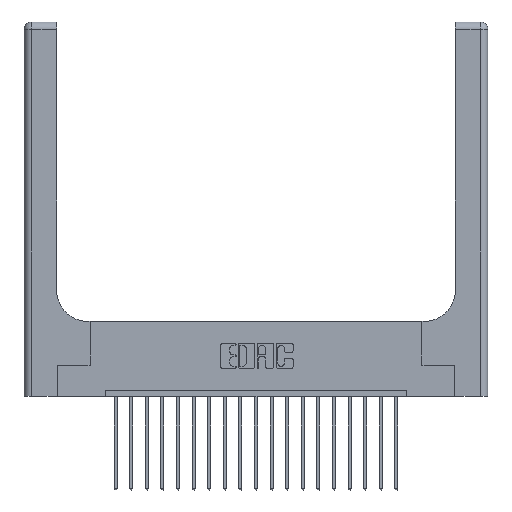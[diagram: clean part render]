
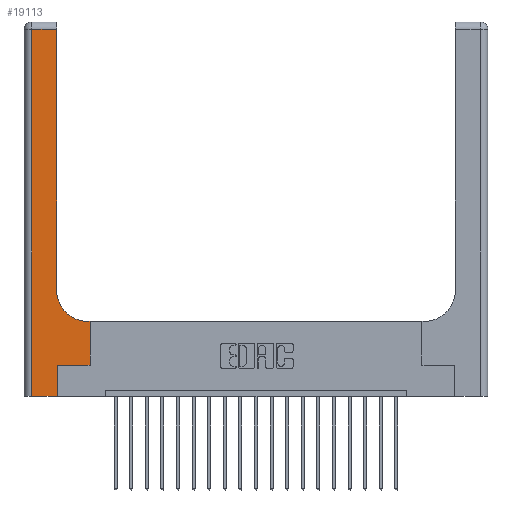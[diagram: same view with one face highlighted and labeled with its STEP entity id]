
A CAD part, top view. The second image highlights one B-rep face of the part: STEP entity #19113.
In plain terms, the highlighted planar face has unit normal (0, 0, 1).
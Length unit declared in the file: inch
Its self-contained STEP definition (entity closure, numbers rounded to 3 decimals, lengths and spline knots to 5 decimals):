
#205 = VERTEX_POINT ( 'NONE', #5809 ) ;
#565 = ORIENTED_EDGE ( 'NONE', *, *, #14055, .T. ) ;
#1562 = PLANE ( 'NONE',  #1674 ) ;
#1574 = VERTEX_POINT ( 'NONE', #9446 ) ;
#1597 = ORIENTED_EDGE ( 'NONE', *, *, #5390, .T. ) ;
#1674 = AXIS2_PLACEMENT_3D ( 'NONE', #18800, #18998, #10796 ) ;
#1866 = VERTEX_POINT ( 'NONE', #15172 ) ;
#1882 = CARTESIAN_POINT ( 'NONE',  ( 0.26, 3., 0.37 ) ) ;
#1920 = CARTESIAN_POINT ( 'NONE',  ( 0.06, 3., 0.37 ) ) ;
#2401 = DIRECTION ( 'NONE',  ( 1., 0., 0. ) ) ;
#2470 = EDGE_CURVE ( 'NONE', #205, #1574, #20418, .T. ) ;
#2886 = CARTESIAN_POINT ( 'NONE',  ( 0.26, 2.94, 0.37 ) ) ;
#4099 = ORIENTED_EDGE ( 'NONE', *, *, #5455, .T. ) ;
#4237 = VECTOR ( 'NONE', #11684, 39.37008 ) ;
#4964 = CARTESIAN_POINT ( 'NONE',  ( 0.265, 0., 0.37 ) ) ;
#5390 = EDGE_CURVE ( 'NONE', #12642, #20198, #8114, .T. ) ;
#5455 = EDGE_CURVE ( 'NONE', #1574, #1866, #7078, .T. ) ;
#5692 = VECTOR ( 'NONE', #7021, 39.37008 ) ;
#5809 = CARTESIAN_POINT ( 'NONE',  ( 0.265, 0., 0.37 ) ) ;
#6081 = CARTESIAN_POINT ( 'NONE',  ( 0., 0., 0.37 ) ) ;
#6245 = EDGE_LOOP ( 'NONE', ( #1597, #9969, #10971, #14447, #13088, #4099, #565, #10019, #12078 ) ) ;
#7021 = DIRECTION ( 'NONE',  ( -1., 0., 0. ) ) ;
#7078 = LINE ( 'NONE', #11968, #18723 ) ;
#7241 = CIRCLE ( 'NONE', #13203, 0.25 ) ;
#7631 = LINE ( 'NONE', #6081, #19554 ) ;
#8114 = LINE ( 'NONE', #1882, #10755 ) ;
#9100 = VERTEX_POINT ( 'NONE', #10749 ) ;
#9446 = CARTESIAN_POINT ( 'NONE',  ( 0.265, 0.25, 0.37 ) ) ;
#9497 = DIRECTION ( 'NONE',  ( 0., 1., 0. ) ) ;
#9542 = FACE_OUTER_BOUND ( 'NONE', #6245, .T. ) ;
#9969 = ORIENTED_EDGE ( 'NONE', *, *, #15376, .T. ) ;
#10019 = ORIENTED_EDGE ( 'NONE', *, *, #19463, .T. ) ;
#10209 = VERTEX_POINT ( 'NONE', #19913 ) ;
#10443 = CARTESIAN_POINT ( 'NONE',  ( 0.26, 0.85, 0.37 ) ) ;
#10749 = CARTESIAN_POINT ( 'NONE',  ( 0.528, 0.6, 0.37 ) ) ;
#10755 = VECTOR ( 'NONE', #19226, 39.37008 ) ;
#10796 = DIRECTION ( 'NONE',  ( -1., 0., 0. ) ) ;
#10971 = ORIENTED_EDGE ( 'NONE', *, *, #12906, .T. ) ;
#11016 = VERTEX_POINT ( 'NONE', #13533 ) ;
#11166 = CARTESIAN_POINT ( 'NONE',  ( 0.528, 0.25, 0.37 ) ) ;
#11408 = VECTOR ( 'NONE', #9497, 39.37008 ) ;
#11684 = DIRECTION ( 'NONE',  ( -1., 0., 0. ) ) ;
#11692 = LINE ( 'NONE', #18029, #5692 ) ;
#11968 = CARTESIAN_POINT ( 'NONE',  ( 0.265, 0.25, 0.37 ) ) ;
#12078 = ORIENTED_EDGE ( 'NONE', *, *, #16099, .T. ) ;
#12175 = CARTESIAN_POINT ( 'NONE',  ( 0.51, 0.85, 0.37 ) ) ;
#12642 = VERTEX_POINT ( 'NONE', #10443 ) ;
#12906 = EDGE_CURVE ( 'NONE', #17054, #11016, #19358, .T. ) ;
#13088 = ORIENTED_EDGE ( 'NONE', *, *, #2470, .T. ) ;
#13203 = AXIS2_PLACEMENT_3D ( 'NONE', #12175, #20073, #19972 ) ;
#13252 = CARTESIAN_POINT ( 'NONE',  ( 0., 2.94, 0.37 ) ) ;
#13533 = CARTESIAN_POINT ( 'NONE',  ( 0.06, 0., 0.37 ) ) ;
#13882 = DIRECTION ( 'NONE',  ( 0., 1., 0. ) ) ;
#14055 = EDGE_CURVE ( 'NONE', #1866, #9100, #15648, .T. ) ;
#14447 = ORIENTED_EDGE ( 'NONE', *, *, #18237, .T. ) ;
#15081 = DIRECTION ( 'NONE',  ( 0., -1., 0. ) ) ;
#15172 = CARTESIAN_POINT ( 'NONE',  ( 0.528, 0.25, 0.37 ) ) ;
#15376 = EDGE_CURVE ( 'NONE', #20198, #17054, #18021, .T. ) ;
#15648 = LINE ( 'NONE', #11166, #19151 ) ;
#15838 = CARTESIAN_POINT ( 'NONE',  ( 0.06, 2.94, 0.37 ) ) ;
#16099 = EDGE_CURVE ( 'NONE', #10209, #12642, #7241, .T. ) ;
#16400 = DIRECTION ( 'NONE',  ( 1., 0., 0. ) ) ;
#17054 = VERTEX_POINT ( 'NONE', #15838 ) ;
#18021 = LINE ( 'NONE', #13252, #4237 ) ;
#18029 = CARTESIAN_POINT ( 'NONE',  ( 0.26, 0.6, 0.37 ) ) ;
#18237 = EDGE_CURVE ( 'NONE', #11016, #205, #7631, .T. ) ;
#18723 = VECTOR ( 'NONE', #2401, 39.37008 ) ;
#18800 = CARTESIAN_POINT ( 'NONE',  ( 0., 3., 0.37 ) ) ;
#18998 = DIRECTION ( 'NONE',  ( 0., 0., -1. ) ) ;
#19113 = ADVANCED_FACE ( 'NONE', ( #9542 ), #1562, .F. ) ;
#19151 = VECTOR ( 'NONE', #13882, 39.37008 ) ;
#19226 = DIRECTION ( 'NONE',  ( 0., 1., 0. ) ) ;
#19358 = LINE ( 'NONE', #1920, #20462 ) ;
#19463 = EDGE_CURVE ( 'NONE', #9100, #10209, #11692, .T. ) ;
#19554 = VECTOR ( 'NONE', #16400, 39.37008 ) ;
#19913 = CARTESIAN_POINT ( 'NONE',  ( 0.51, 0.6, 0.37 ) ) ;
#19972 = DIRECTION ( 'NONE',  ( 1., 0., 0. ) ) ;
#20073 = DIRECTION ( 'NONE',  ( 0., 0., -1. ) ) ;
#20198 = VERTEX_POINT ( 'NONE', #2886 ) ;
#20418 = LINE ( 'NONE', #4964, #11408 ) ;
#20462 = VECTOR ( 'NONE', #15081, 39.37008 ) ;
